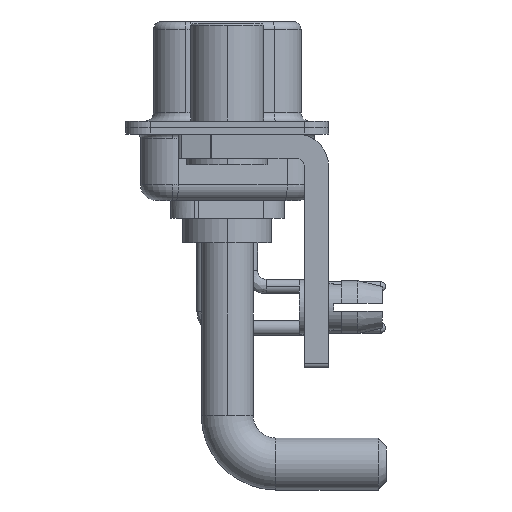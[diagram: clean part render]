
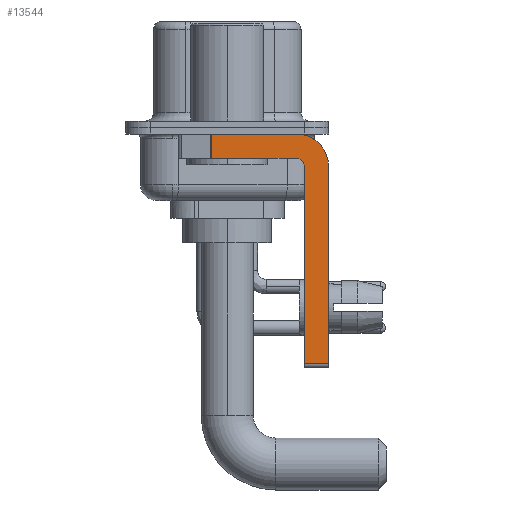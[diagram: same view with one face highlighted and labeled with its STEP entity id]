
A CAD part, left-side view. The second image highlights one B-rep face of the part: STEP entity #13544.
In plain terms, the highlighted planar face has unit normal (-1, 0, 0).
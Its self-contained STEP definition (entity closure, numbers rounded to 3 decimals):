
#1205 = DIRECTION ( 'NONE',  ( 0., -1., 0. ) ) ;
#3038 = CARTESIAN_POINT ( 'NONE',  ( -2.9, -6.25, -2.4 ) ) ;
#3226 = VECTOR ( 'NONE', #1205, 1000. ) ;
#3274 = VERTEX_POINT ( 'NONE', #4164 ) ;
#3278 = LINE ( 'NONE', #26119, #13887 ) ;
#3593 = CARTESIAN_POINT ( 'NONE',  ( -2.9, 0.978, -1.9 ) ) ;
#3982 = CARTESIAN_POINT ( 'NONE',  ( -2.9, -4.75, -14.55 ) ) ;
#4164 = CARTESIAN_POINT ( 'NONE',  ( -2.9, 0.978, -0.4 ) ) ;
#4409 = VERTEX_POINT ( 'NONE', #3593 ) ;
#5280 = PLANE ( 'NONE',  #11235 ) ;
#5331 = VERTEX_POINT ( 'NONE', #21358 ) ;
#5982 = CARTESIAN_POINT ( 'NONE',  ( -2.9, -4.25, -14.55 ) ) ;
#6363 = EDGE_CURVE ( 'NONE', #3274, #7883, #22853, .T. ) ;
#6533 = ORIENTED_EDGE ( 'NONE', *, *, #11361, .F. ) ;
#6978 = VECTOR ( 'NONE', #23002, 1000. ) ;
#7370 = CARTESIAN_POINT ( 'NONE',  ( -2.9, -4.25, -1.9 ) ) ;
#7883 = VERTEX_POINT ( 'NONE', #32402 ) ;
#8143 = ORIENTED_EDGE ( 'NONE', *, *, #11936, .T. ) ;
#8342 = EDGE_CURVE ( 'NONE', #7883, #24195, #20040, .T. ) ;
#8973 = VECTOR ( 'NONE', #20417, 1000. ) ;
#9021 = EDGE_CURVE ( 'NONE', #3274, #4409, #18238, .T. ) ;
#9886 = EDGE_CURVE ( 'NONE', #5331, #29998, #27501, .T. ) ;
#9925 = CARTESIAN_POINT ( 'NONE',  ( -2.9, -4.25, -1.9 ) ) ;
#10256 = CARTESIAN_POINT ( 'NONE',  ( -2.9, 3., -0.4 ) ) ;
#11142 = CARTESIAN_POINT ( 'NONE',  ( -2.9, -4.75, -14.8 ) ) ;
#11235 = AXIS2_PLACEMENT_3D ( 'NONE', #22829, #15051, #30575 ) ;
#11361 = EDGE_CURVE ( 'NONE', #11901, #5331, #31320, .T. ) ;
#11363 = DIRECTION ( 'NONE',  ( 1., 0., 0. ) ) ;
#11901 = VERTEX_POINT ( 'NONE', #3982 ) ;
#11936 = EDGE_CURVE ( 'NONE', #11901, #32278, #23848, .T. ) ;
#13091 = ORIENTED_EDGE ( 'NONE', *, *, #6363, .F. ) ;
#13128 = DIRECTION ( 'NONE',  ( 0., 0., 1. ) ) ;
#13544 = ADVANCED_FACE ( 'NONE', ( #20189 ), #5280, .F. ) ;
#13669 = EDGE_CURVE ( 'NONE', #24195, #32278, #3278, .T. ) ;
#13887 = VECTOR ( 'NONE', #26286, 1000. ) ;
#14495 = CARTESIAN_POINT ( 'NONE',  ( -2.9, -6.25, -14.55 ) ) ;
#15051 = DIRECTION ( 'NONE',  ( 1., 0., 0. ) ) ;
#15446 = VECTOR ( 'NONE', #18763, 1000. ) ;
#15658 = EDGE_CURVE ( 'NONE', #29998, #4409, #30356, .T. ) ;
#17156 = CARTESIAN_POINT ( 'NONE',  ( -2.9, -4.25, -2.4 ) ) ;
#18238 = LINE ( 'NONE', #30812, #8973 ) ;
#18763 = DIRECTION ( 'NONE',  ( 0., 0., 1. ) ) ;
#18942 = EDGE_LOOP ( 'NONE', ( #13091, #25889, #28157, #26001, #6533, #8143, #28626, #31463 ) ) ;
#20040 = CIRCLE ( 'NONE', #24269, 2. ) ;
#20109 = DIRECTION ( 'NONE',  ( -1., 0., 0. ) ) ;
#20189 = FACE_OUTER_BOUND ( 'NONE', #18942, .T. ) ;
#20417 = DIRECTION ( 'NONE',  ( 0., 0., -1. ) ) ;
#21358 = CARTESIAN_POINT ( 'NONE',  ( -2.9, -4.75, -2.4 ) ) ;
#22829 = CARTESIAN_POINT ( 'NONE',  ( -2.9, -4.25, -2.4 ) ) ;
#22853 = LINE ( 'NONE', #10256, #6978 ) ;
#23002 = DIRECTION ( 'NONE',  ( 0., -1., 0. ) ) ;
#23848 = LINE ( 'NONE', #5982, #3226 ) ;
#24195 = VERTEX_POINT ( 'NONE', #3038 ) ;
#24269 = AXIS2_PLACEMENT_3D ( 'NONE', #17156, #11363, #27261 ) ;
#25253 = DIRECTION ( 'NONE',  ( 0., 1., 0. ) ) ;
#25610 = VECTOR ( 'NONE', #25253, 1000. ) ;
#25889 = ORIENTED_EDGE ( 'NONE', *, *, #9021, .T. ) ;
#25916 = AXIS2_PLACEMENT_3D ( 'NONE', #27874, #20109, #13128 ) ;
#26001 = ORIENTED_EDGE ( 'NONE', *, *, #9886, .F. ) ;
#26119 = CARTESIAN_POINT ( 'NONE',  ( -2.9, -6.25, -2.4 ) ) ;
#26286 = DIRECTION ( 'NONE',  ( 0., 0., -1. ) ) ;
#27261 = DIRECTION ( 'NONE',  ( 0., 0., -1. ) ) ;
#27501 = CIRCLE ( 'NONE', #25916, 0.5 ) ;
#27874 = CARTESIAN_POINT ( 'NONE',  ( -2.9, -4.25, -2.4 ) ) ;
#28157 = ORIENTED_EDGE ( 'NONE', *, *, #15658, .F. ) ;
#28626 = ORIENTED_EDGE ( 'NONE', *, *, #13669, .F. ) ;
#29998 = VERTEX_POINT ( 'NONE', #9925 ) ;
#30356 = LINE ( 'NONE', #7370, #25610 ) ;
#30575 = DIRECTION ( 'NONE',  ( 0., 0., -1. ) ) ;
#30812 = CARTESIAN_POINT ( 'NONE',  ( -2.9, 0.978, -1.9 ) ) ;
#31320 = LINE ( 'NONE', #11142, #15446 ) ;
#31463 = ORIENTED_EDGE ( 'NONE', *, *, #8342, .F. ) ;
#32278 = VERTEX_POINT ( 'NONE', #14495 ) ;
#32402 = CARTESIAN_POINT ( 'NONE',  ( -2.9, -4.25, -0.4 ) ) ;
